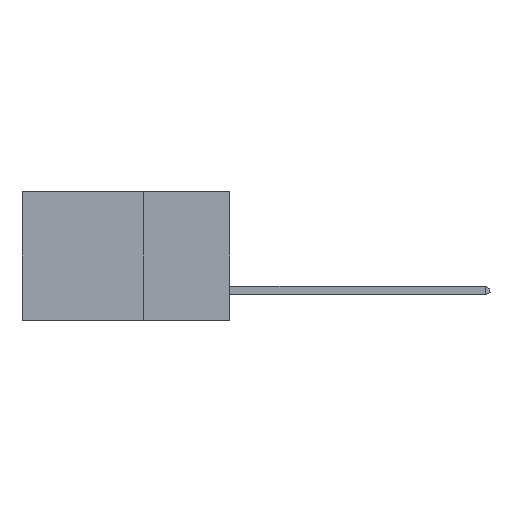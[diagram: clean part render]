
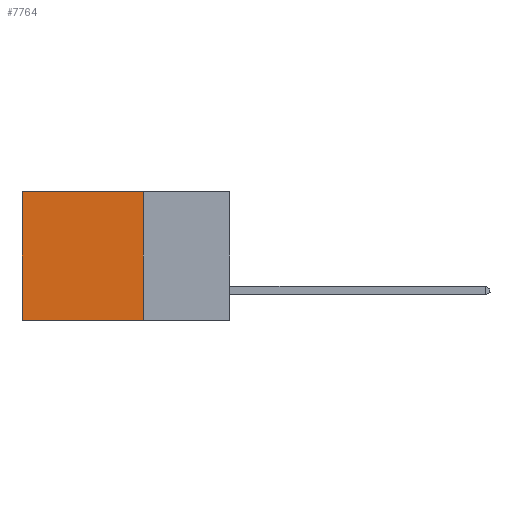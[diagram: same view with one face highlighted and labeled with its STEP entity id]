
A CAD part, left-side view. The second image highlights one B-rep face of the part: STEP entity #7764.
In plain terms, the highlighted planar face has unit normal (-1, 0, 0).
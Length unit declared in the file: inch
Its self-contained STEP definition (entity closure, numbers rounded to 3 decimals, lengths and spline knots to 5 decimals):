
#269 = CARTESIAN_POINT ( 'NONE',  ( 0.298, 0.25, 0. ) ) ;
#519 = EDGE_CURVE ( 'NONE', #5607, #4708, #10932, .T. ) ;
#535 = CARTESIAN_POINT ( 'NONE',  ( 0.298, 0.25, 0. ) ) ;
#1370 = CARTESIAN_POINT ( 'NONE',  ( 0.298, 0.25, -0.37 ) ) ;
#2563 = EDGE_CURVE ( 'NONE', #5607, #7103, #15928, .T. ) ;
#2701 = DIRECTION ( 'NONE',  ( 0., 1., 0. ) ) ;
#3248 = DIRECTION ( 'NONE',  ( 0., 0., -1. ) ) ;
#3534 = EDGE_CURVE ( 'NONE', #7103, #7844, #7352, .T. ) ;
#3988 = VECTOR ( 'NONE', #2701, 39.37008 ) ;
#4229 = DIRECTION ( 'NONE',  ( 1., 0., 0. ) ) ;
#4248 = ORIENTED_EDGE ( 'NONE', *, *, #10979, .T. ) ;
#4282 = PLANE ( 'NONE',  #16098 ) ;
#4481 = EDGE_LOOP ( 'NONE', ( #4248, #4827, #7176, #6054 ) ) ;
#4708 = VERTEX_POINT ( 'NONE', #7478 ) ;
#4827 = ORIENTED_EDGE ( 'NONE', *, *, #3534, .F. ) ;
#5423 = CARTESIAN_POINT ( 'NONE',  ( 0.298, 0.25, -0.37 ) ) ;
#5607 = VERTEX_POINT ( 'NONE', #15969 ) ;
#5662 = CARTESIAN_POINT ( 'NONE',  ( 0.298, 0.25, 0. ) ) ;
#5907 = DIRECTION ( 'NONE',  ( 0., 0., -1. ) ) ;
#5913 = VECTOR ( 'NONE', #3248, 39.37008 ) ;
#6054 = ORIENTED_EDGE ( 'NONE', *, *, #519, .T. ) ;
#7103 = VERTEX_POINT ( 'NONE', #5423 ) ;
#7161 = VECTOR ( 'NONE', #5907, 39.37008 ) ;
#7176 = ORIENTED_EDGE ( 'NONE', *, *, #2563, .F. ) ;
#7352 = LINE ( 'NONE', #1370, #3988 ) ;
#7478 = CARTESIAN_POINT ( 'NONE',  ( 0.298, 0.6, 0. ) ) ;
#7764 = ADVANCED_FACE ( 'NONE', ( #14877 ), #4282, .F. ) ;
#7844 = VERTEX_POINT ( 'NONE', #8197 ) ;
#8045 = DIRECTION ( 'NONE',  ( 0., 0., -1. ) ) ;
#8197 = CARTESIAN_POINT ( 'NONE',  ( 0.298, 0.6, -0.37 ) ) ;
#8267 = CARTESIAN_POINT ( 'NONE',  ( 0.298, 0.6, 0. ) ) ;
#10932 = LINE ( 'NONE', #269, #12285 ) ;
#10979 = EDGE_CURVE ( 'NONE', #4708, #7844, #12655, .T. ) ;
#12285 = VECTOR ( 'NONE', #15463, 39.37008 ) ;
#12655 = LINE ( 'NONE', #8267, #7161 ) ;
#14877 = FACE_OUTER_BOUND ( 'NONE', #4481, .T. ) ;
#15463 = DIRECTION ( 'NONE',  ( 0., 1., 0. ) ) ;
#15928 = LINE ( 'NONE', #535, #5913 ) ;
#15969 = CARTESIAN_POINT ( 'NONE',  ( 0.298, 0.25, 0. ) ) ;
#16098 = AXIS2_PLACEMENT_3D ( 'NONE', #5662, #4229, #8045 ) ;
